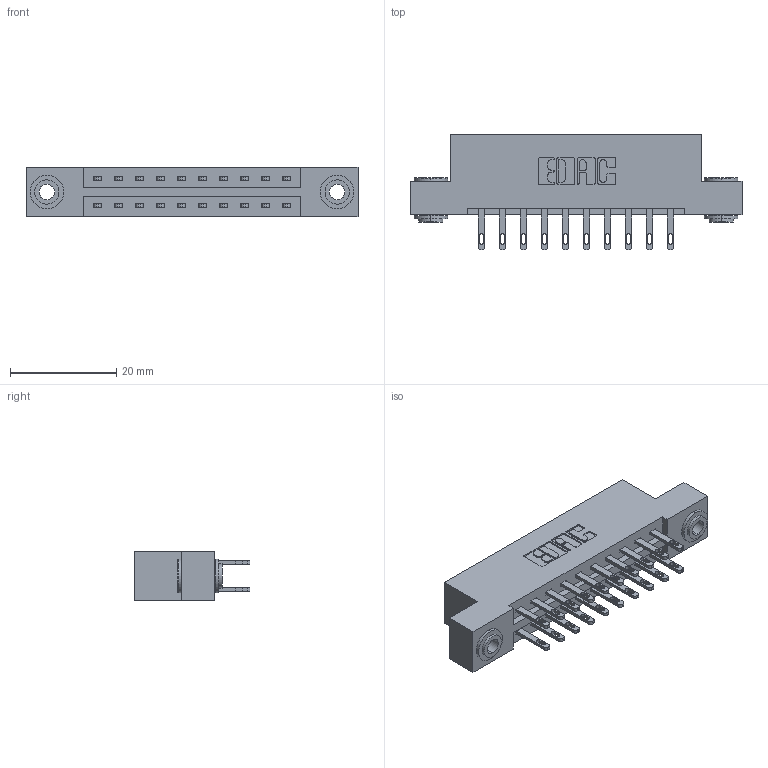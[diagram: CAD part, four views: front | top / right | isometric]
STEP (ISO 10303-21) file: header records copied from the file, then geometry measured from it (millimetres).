
FILE_DESCRIPTION (( 'STEP AP203' ), '1' );
FILE_NAME ('337-020-500-203.STEP', '2019-10-08T13:40:16', ( '' ), ( '' ), 'SwSTEP 2.0', 'SolidWorks 2016', '' );
FILE_SCHEMA (( 'CONFIG_CONTROL_DESIGN' ));
Length unit declared in the file: inch
Products named in the file (4): 345-250-002_345-250-002-102; 337 Part_Flush Mounting Lugs - 0.156 Dia-TH; 337-020-500-203; 345-292-001_345-293-100
Assembly tree (23 placements, depth 2):
  337-020-500-203
    337 Part_Flush Mounting Lugs - 0.156 Dia-TH
    345-292-001_345-293-100  x20
    345-250-002_345-250-002-102  x2
Bounding box: 62.64 x 21.85 x 9.4 mm (x, y, z)
Volume: 6255.7 mm3; surface area: 7207.5 mm2
Topology: 23 solids, 23 shells, 1152 faces, 3447 edges, 2294 vertices
Faces by surface type: plane 720, cylinder 424, cone 8
Entity records: 12472 total; most frequent: CARTESIAN_POINT 2101, ORIENTED_EDGE 2030, DIRECTION 1881, EDGE_CURVE 1015, VECTOR 859, LINE 859, VERTEX_POINT 674, AXIS2_PLACEMENT_3D 511
